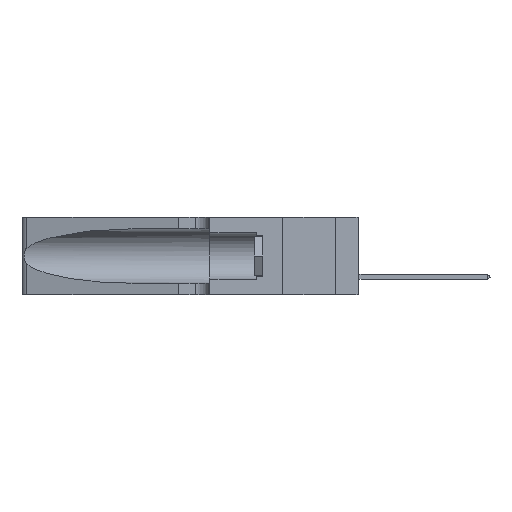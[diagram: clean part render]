
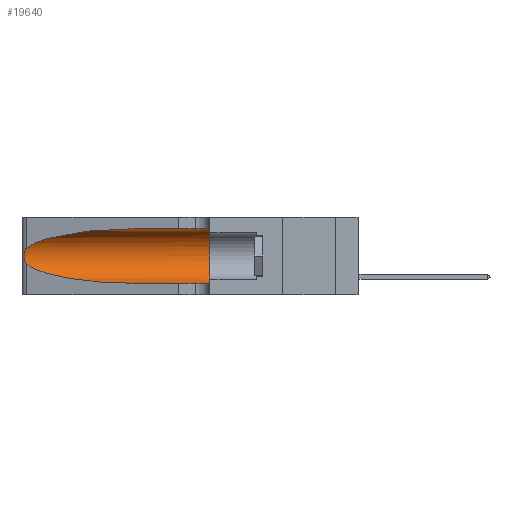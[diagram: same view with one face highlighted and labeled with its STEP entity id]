
A CAD part, left-side view. The second image highlights one B-rep face of the part: STEP entity #19640.
In plain terms, the highlighted cylindrical face has radius 3.308 mm (diameter 6.617 mm), a partial arc.
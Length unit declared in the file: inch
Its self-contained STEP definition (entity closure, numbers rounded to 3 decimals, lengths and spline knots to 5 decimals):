
#270 = CARTESIAN_POINT ( 'NONE',  ( 0.26075, 1.23896, 0.19203 ) ) ;
#478 = CARTESIAN_POINT ( 'NONE',  ( 0.25856, 1.23593, 0.16098 ) ) ;
#1163 = VERTEX_POINT ( 'NONE', #18319 ) ;
#1390 =( BOUNDED_CURVE ( )  B_SPLINE_CURVE ( 3, ( #21336, #19783, #12974, #14730 ),
 .UNSPECIFIED., .F., .F. ) 
 B_SPLINE_CURVE_WITH_KNOTS ( ( 4, 4 ),
 ( 1.5708, 2.84003 ),
 .UNSPECIFIED. ) 
 CURVE ( )  GEOMETRIC_REPRESENTATION_ITEM ( )  RATIONAL_B_SPLINE_CURVE ( ( 1., 0.87, 0.87, 1. ) ) 
 REPRESENTATION_ITEM ( '' )  );
#1709 = VERTEX_POINT ( 'NONE', #4563 ) ;
#2019 = ORIENTED_EDGE ( 'NONE', *, *, #11122, .T. ) ;
#2791 = DIRECTION ( 'NONE',  ( 0., 0., 1. ) ) ;
#2962 = LINE ( 'NONE', #20380, #9930 ) ;
#3197 = CARTESIAN_POINT ( 'NONE',  ( 0.1305, 0.72297, 0.05475 ) ) ;
#3593 = CIRCLE ( 'NONE', #12984, 0.13025 ) ;
#3760 = CARTESIAN_POINT ( 'NONE',  ( 0.25639, 1.23184, 0.21858 ) ) ;
#4053 = CARTESIAN_POINT ( 'NONE',  ( 0.26017, 1.23833, 0.17102 ) ) ;
#4563 = CARTESIAN_POINT ( 'NONE',  ( 0.1305, 0.35, 0.05475 ) ) ;
#4710 = ORIENTED_EDGE ( 'NONE', *, *, #6913, .T. ) ;
#4872 = AXIS2_PLACEMENT_3D ( 'NONE', #15278, #10041, #6764 ) ;
#5188 = CARTESIAN_POINT ( 'NONE',  ( 0.1305, 1.61858, 0.31525 ) ) ;
#5250 = CYLINDRICAL_SURFACE ( 'NONE', #4872, 0.13025 ) ;
#5651 = CARTESIAN_POINT ( 'NONE',  ( 0.25789, 1.23486, 0.15765 ) ) ;
#6099 =( BOUNDED_CURVE ( )  B_SPLINE_CURVE ( 3, ( #12468, #15715, #10828, #3197 ),
 .UNSPECIFIED., .F., .T. ) 
 B_SPLINE_CURVE_WITH_KNOTS ( ( 4, 4 ),
 ( 3.44316, 4.71239 ),
 .UNSPECIFIED. ) 
 CURVE ( )  GEOMETRIC_REPRESENTATION_ITEM ( )  RATIONAL_B_SPLINE_CURVE ( ( 1., 0.87, 0.87, 1. ) ) 
 REPRESENTATION_ITEM ( '' )  );
#6470 = EDGE_CURVE ( 'NONE', #18114, #1163, #7968, .T. ) ;
#6764 = DIRECTION ( 'NONE',  ( 0., 0., -1. ) ) ;
#6913 = EDGE_CURVE ( 'NONE', #14436, #18776, #6099, .T. ) ;
#7056 = DIRECTION ( 'NONE',  ( 0., -1., 0. ) ) ;
#7167 = EDGE_CURVE ( 'NONE', #18114, #10087, #1390, .T. ) ;
#7278 = EDGE_LOOP ( 'NONE', ( #12772, #17072, #4710, #2019, #15372, #7697 ) ) ;
#7378 = CARTESIAN_POINT ( 'NONE',  ( 0.25854, 1.2359, 0.20912 ) ) ;
#7523 = CARTESIAN_POINT ( 'NONE',  ( 0.25555, 1.22993, 0.14849 ) ) ;
#7697 = ORIENTED_EDGE ( 'NONE', *, *, #6470, .F. ) ;
#7968 = LINE ( 'NONE', #5188, #18140 ) ;
#8152 = CARTESIAN_POINT ( 'NONE',  ( 0.1305, 0.35, 0.185 ) ) ;
#9119 = B_SPLINE_CURVE_WITH_KNOTS ( 'NONE', 3,
 ( #17196, #10379, #3760, #10803, #7378, #17613, #270, #12584, #4053, #478, #5651, #19399, #7523, #15901 ),
 .UNSPECIFIED., .F., .F.,
 ( 4, 2, 2, 2, 2, 2, 4 ),
 ( 0., 0.00027, 0.00053, 0.00107, 0.0016, 0.00187, 0.00214 ),
 .UNSPECIFIED. ) ;
#9930 = VECTOR ( 'NONE', #7056, 39.37008 ) ;
#10041 = DIRECTION ( 'NONE',  ( 0., -1., 0. ) ) ;
#10087 = VERTEX_POINT ( 'NONE', #12620 ) ;
#10319 = CARTESIAN_POINT ( 'NONE',  ( 0.25487, 1.22718, 0.14631 ) ) ;
#10379 = CARTESIAN_POINT ( 'NONE',  ( 0.25555, 1.22994, 0.2215 ) ) ;
#10656 = CARTESIAN_POINT ( 'NONE',  ( 0.1305, 0.72297, 0.05475 ) ) ;
#10803 = CARTESIAN_POINT ( 'NONE',  ( 0.25787, 1.23484, 0.2124 ) ) ;
#10828 = CARTESIAN_POINT ( 'NONE',  ( 0.18966, 0.96281, 0.05475 ) ) ;
#11122 = EDGE_CURVE ( 'NONE', #18776, #1709, #2962, .T. ) ;
#12468 = CARTESIAN_POINT ( 'NONE',  ( 0.25487, 1.22718, 0.14631 ) ) ;
#12584 = CARTESIAN_POINT ( 'NONE',  ( 0.26075, 1.23896, 0.178 ) ) ;
#12620 = CARTESIAN_POINT ( 'NONE',  ( 0.25487, 1.22718, 0.22369 ) ) ;
#12772 = ORIENTED_EDGE ( 'NONE', *, *, #7167, .T. ) ;
#12974 = CARTESIAN_POINT ( 'NONE',  ( 0.2373, 1.15595, 0.28018 ) ) ;
#12984 = AXIS2_PLACEMENT_3D ( 'NONE', #8152, #18232, #2791 ) ;
#14436 = VERTEX_POINT ( 'NONE', #10319 ) ;
#14730 = CARTESIAN_POINT ( 'NONE',  ( 0.25487, 1.22718, 0.22369 ) ) ;
#14833 = EDGE_CURVE ( 'NONE', #1163, #1709, #3593, .T. ) ;
#15278 = CARTESIAN_POINT ( 'NONE',  ( 0.1305, 1.61858, 0.185 ) ) ;
#15372 = ORIENTED_EDGE ( 'NONE', *, *, #14833, .F. ) ;
#15465 = DIRECTION ( 'NONE',  ( 0., -1., 0. ) ) ;
#15715 = CARTESIAN_POINT ( 'NONE',  ( 0.2373, 1.15595, 0.08982 ) ) ;
#15901 = CARTESIAN_POINT ( 'NONE',  ( 0.25487, 1.22718, 0.14631 ) ) ;
#17072 = ORIENTED_EDGE ( 'NONE', *, *, #20434, .T. ) ;
#17196 = CARTESIAN_POINT ( 'NONE',  ( 0.25487, 1.22718, 0.22369 ) ) ;
#17613 = CARTESIAN_POINT ( 'NONE',  ( 0.26018, 1.23835, 0.19895 ) ) ;
#18114 = VERTEX_POINT ( 'NONE', #19349 ) ;
#18140 = VECTOR ( 'NONE', #15465, 39.37008 ) ;
#18232 = DIRECTION ( 'NONE',  ( 0., 1., 0. ) ) ;
#18319 = CARTESIAN_POINT ( 'NONE',  ( 0.1305, 0.35, 0.31525 ) ) ;
#18776 = VERTEX_POINT ( 'NONE', #10656 ) ;
#19349 = CARTESIAN_POINT ( 'NONE',  ( 0.1305, 0.72297, 0.31525 ) ) ;
#19399 = CARTESIAN_POINT ( 'NONE',  ( 0.25639, 1.23186, 0.15144 ) ) ;
#19640 = ADVANCED_FACE ( 'NONE', ( #20986 ), #5250, .F. ) ;
#19783 = CARTESIAN_POINT ( 'NONE',  ( 0.18966, 0.96281, 0.31525 ) ) ;
#20380 = CARTESIAN_POINT ( 'NONE',  ( 0.1305, 1.61858, 0.05475 ) ) ;
#20434 = EDGE_CURVE ( 'NONE', #10087, #14436, #9119, .T. ) ;
#20986 = FACE_OUTER_BOUND ( 'NONE', #7278, .T. ) ;
#21336 = CARTESIAN_POINT ( 'NONE',  ( 0.1305, 0.72297, 0.31525 ) ) ;
